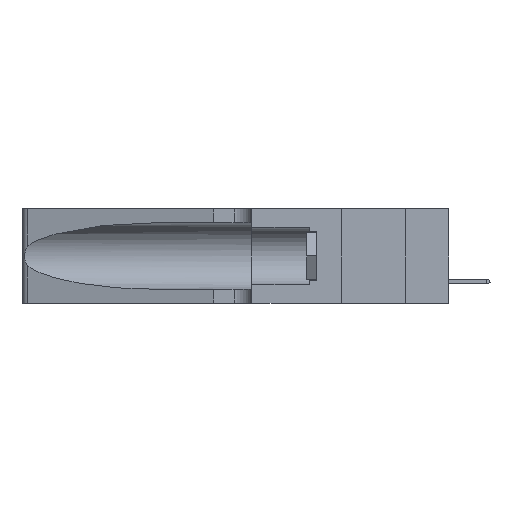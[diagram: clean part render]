
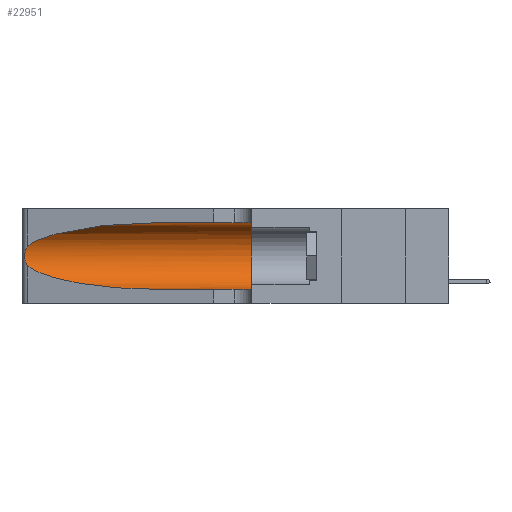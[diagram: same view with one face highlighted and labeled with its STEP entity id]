
A CAD part, left-side view. The second image highlights one B-rep face of the part: STEP entity #22951.
In plain terms, the highlighted cylindrical face has radius 3.308 mm (diameter 6.617 mm), a partial arc.
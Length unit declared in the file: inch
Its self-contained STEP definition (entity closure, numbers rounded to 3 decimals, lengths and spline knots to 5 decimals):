
#94 = AXIS2_PLACEMENT_3D ( 'NONE', #29625, #13818, #10148 ) ;
#668 = CARTESIAN_POINT ( 'NONE',  ( 0.26018, 1.23835, 0.19895 ) ) ;
#1257 = CARTESIAN_POINT ( 'NONE',  ( 0.1305, 0.35, 0.05475 ) ) ;
#1438 = CARTESIAN_POINT ( 'NONE',  ( 0.25487, 1.22718, 0.22369 ) ) ;
#1681 = CARTESIAN_POINT ( 'NONE',  ( 0.25856, 1.23593, 0.16098 ) ) ;
#2396 = LINE ( 'NONE', #33065, #23196 ) ;
#3825 = CARTESIAN_POINT ( 'NONE',  ( 0.25787, 1.23484, 0.2124 ) ) ;
#4539 = CARTESIAN_POINT ( 'NONE',  ( 0.26075, 1.23896, 0.19203 ) ) ;
#4835 = CARTESIAN_POINT ( 'NONE',  ( 0.25639, 1.23186, 0.15144 ) ) ;
#5126 = VERTEX_POINT ( 'NONE', #14387 ) ;
#5856 = CARTESIAN_POINT ( 'NONE',  ( 0.25555, 1.22993, 0.14849 ) ) ;
#6302 = EDGE_LOOP ( 'NONE', ( #36476, #41491, #7455, #27327, #18211, #40297 ) ) ;
#6393 = CARTESIAN_POINT ( 'NONE',  ( 0.2373, 1.15595, 0.08982 ) ) ;
#6638 = CARTESIAN_POINT ( 'NONE',  ( 0.1305, 0.72297, 0.05475 ) ) ;
#6682 = VERTEX_POINT ( 'NONE', #1257 ) ;
#7455 = ORIENTED_EDGE ( 'NONE', *, *, #13772, .T. ) ;
#7792 = CARTESIAN_POINT ( 'NONE',  ( 0.26075, 1.23896, 0.178 ) ) ;
#8381 = CARTESIAN_POINT ( 'NONE',  ( 0.25789, 1.23486, 0.15765 ) ) ;
#9141 = CARTESIAN_POINT ( 'NONE',  ( 0.1305, 0.35, 0.185 ) ) ;
#9488 = VECTOR ( 'NONE', #21736, 39.37008 ) ;
#10148 = DIRECTION ( 'NONE',  ( 0., 0., -1. ) ) ;
#11848 = CARTESIAN_POINT ( 'NONE',  ( 0.2373, 1.15595, 0.28018 ) ) ;
#12010 = CARTESIAN_POINT ( 'NONE',  ( 0.25487, 1.22718, 0.14631 ) ) ;
#12681 = DIRECTION ( 'NONE',  ( 0., 0., 1. ) ) ;
#13709 = CARTESIAN_POINT ( 'NONE',  ( 0.26017, 1.23833, 0.17102 ) ) ;
#13772 = EDGE_CURVE ( 'NONE', #27777, #28672, #31182, .T. ) ;
#13818 = DIRECTION ( 'NONE',  ( 0., -1., 0. ) ) ;
#14387 = CARTESIAN_POINT ( 'NONE',  ( 0.1305, 0.72297, 0.31525 ) ) ;
#14730 = CARTESIAN_POINT ( 'NONE',  ( 0.1305, 0.72297, 0.05475 ) ) ;
#17118 = EDGE_CURVE ( 'NONE', #22447, #27777, #26269, .T. ) ;
#18083 = LINE ( 'NONE', #37588, #9488 ) ;
#18211 = ORIENTED_EDGE ( 'NONE', *, *, #28793, .F. ) ;
#19352 = VERTEX_POINT ( 'NONE', #24409 ) ;
#19667 = CIRCLE ( 'NONE', #21992, 0.13025 ) ;
#21736 = DIRECTION ( 'NONE',  ( 0., -1., 0. ) ) ;
#21992 = AXIS2_PLACEMENT_3D ( 'NONE', #9141, #32144, #12681 ) ;
#22220 = CARTESIAN_POINT ( 'NONE',  ( 0.25487, 1.22718, 0.22369 ) ) ;
#22447 = VERTEX_POINT ( 'NONE', #1438 ) ;
#22578 = CARTESIAN_POINT ( 'NONE',  ( 0.25487, 1.22718, 0.14631 ) ) ;
#22916 = EDGE_CURVE ( 'NONE', #5126, #19352, #2396, .T. ) ;
#22951 = ADVANCED_FACE ( 'NONE', ( #31846 ), #28296, .F. ) ;
#23196 = VECTOR ( 'NONE', #29757, 39.37008 ) ;
#23497 = EDGE_CURVE ( 'NONE', #28672, #6682, #18083, .T. ) ;
#24409 = CARTESIAN_POINT ( 'NONE',  ( 0.1305, 0.35, 0.31525 ) ) ;
#25284 = CARTESIAN_POINT ( 'NONE',  ( 0.18966, 0.96281, 0.31525 ) ) ;
#25542 =( BOUNDED_CURVE ( )  B_SPLINE_CURVE ( 3, ( #31486, #25284, #11848, #38256 ),
 .UNSPECIFIED., .F., .F. ) 
 B_SPLINE_CURVE_WITH_KNOTS ( ( 4, 4 ),
 ( 1.5708, 2.84003 ),
 .UNSPECIFIED. ) 
 CURVE ( )  GEOMETRIC_REPRESENTATION_ITEM ( )  RATIONAL_B_SPLINE_CURVE ( ( 1., 0.87, 0.87, 1. ) ) 
 REPRESENTATION_ITEM ( '' )  );
#26269 = B_SPLINE_CURVE_WITH_KNOTS ( 'NONE', 3,
 ( #22220, #29027, #32835, #3825, #26582, #668, #4539, #7792, #13709, #1681, #8381, #4835, #5856, #29371 ),
 .UNSPECIFIED., .F., .F.,
 ( 4, 2, 2, 2, 2, 2, 4 ),
 ( 0., 0.00027, 0.00053, 0.00107, 0.0016, 0.00187, 0.00214 ),
 .UNSPECIFIED. ) ;
#26582 = CARTESIAN_POINT ( 'NONE',  ( 0.25854, 1.2359, 0.20912 ) ) ;
#27327 = ORIENTED_EDGE ( 'NONE', *, *, #23497, .T. ) ;
#27777 = VERTEX_POINT ( 'NONE', #12010 ) ;
#28296 = CYLINDRICAL_SURFACE ( 'NONE', #94, 0.13025 ) ;
#28672 = VERTEX_POINT ( 'NONE', #14730 ) ;
#28793 = EDGE_CURVE ( 'NONE', #19352, #6682, #19667, .T. ) ;
#29027 = CARTESIAN_POINT ( 'NONE',  ( 0.25555, 1.22994, 0.2215 ) ) ;
#29371 = CARTESIAN_POINT ( 'NONE',  ( 0.25487, 1.22718, 0.14631 ) ) ;
#29625 = CARTESIAN_POINT ( 'NONE',  ( 0.1305, 1.61858, 0.185 ) ) ;
#29757 = DIRECTION ( 'NONE',  ( 0., -1., 0. ) ) ;
#29931 = EDGE_CURVE ( 'NONE', #5126, #22447, #25542, .T. ) ;
#31182 =( BOUNDED_CURVE ( )  B_SPLINE_CURVE ( 3, ( #22578, #6393, #35471, #6638 ),
 .UNSPECIFIED., .F., .F. ) 
 B_SPLINE_CURVE_WITH_KNOTS ( ( 4, 4 ),
 ( 3.44316, 4.71239 ),
 .UNSPECIFIED. ) 
 CURVE ( )  GEOMETRIC_REPRESENTATION_ITEM ( )  RATIONAL_B_SPLINE_CURVE ( ( 1., 0.87, 0.87, 1. ) ) 
 REPRESENTATION_ITEM ( '' )  );
#31486 = CARTESIAN_POINT ( 'NONE',  ( 0.1305, 0.72297, 0.31525 ) ) ;
#31846 = FACE_OUTER_BOUND ( 'NONE', #6302, .T. ) ;
#32144 = DIRECTION ( 'NONE',  ( 0., 1., 0. ) ) ;
#32835 = CARTESIAN_POINT ( 'NONE',  ( 0.25639, 1.23184, 0.21858 ) ) ;
#33065 = CARTESIAN_POINT ( 'NONE',  ( 0.1305, 1.61858, 0.31525 ) ) ;
#35471 = CARTESIAN_POINT ( 'NONE',  ( 0.18966, 0.96281, 0.05475 ) ) ;
#36476 = ORIENTED_EDGE ( 'NONE', *, *, #29931, .T. ) ;
#37588 = CARTESIAN_POINT ( 'NONE',  ( 0.1305, 1.61858, 0.05475 ) ) ;
#38256 = CARTESIAN_POINT ( 'NONE',  ( 0.25487, 1.22718, 0.22369 ) ) ;
#40297 = ORIENTED_EDGE ( 'NONE', *, *, #22916, .F. ) ;
#41491 = ORIENTED_EDGE ( 'NONE', *, *, #17118, .T. ) ;
